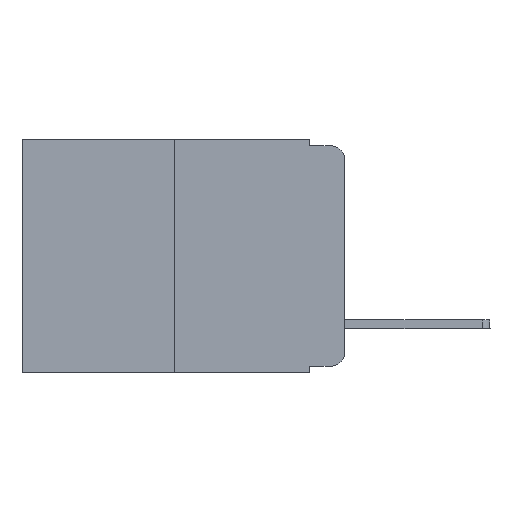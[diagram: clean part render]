
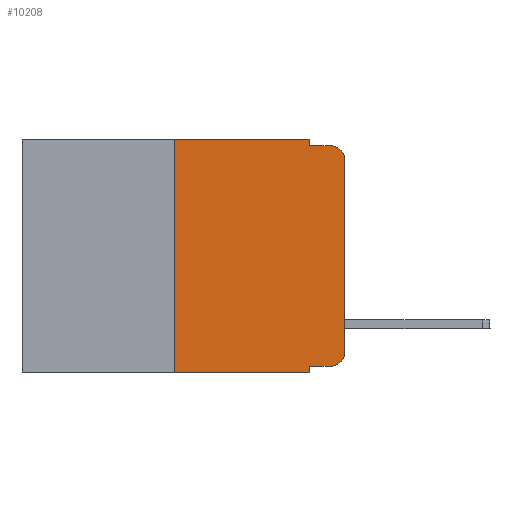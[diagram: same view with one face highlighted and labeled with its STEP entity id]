
A CAD part, left-side view. The second image highlights one B-rep face of the part: STEP entity #10208.
In plain terms, the highlighted planar face has unit normal (-1, 0, 0).
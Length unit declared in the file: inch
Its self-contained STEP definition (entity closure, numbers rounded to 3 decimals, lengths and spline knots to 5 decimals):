
#117 = ORIENTED_EDGE ( 'NONE', *, *, #11305, .F. ) ;
#152 = EDGE_CURVE ( 'NONE', #15001, #13935, #11804, .T. ) ;
#544 = DIRECTION ( 'NONE',  ( 1., 0., 0. ) ) ;
#600 = VECTOR ( 'NONE', #2760, 39.37008 ) ;
#663 = LINE ( 'NONE', #4531, #10908 ) ;
#776 = DIRECTION ( 'NONE',  ( 0., 0., -1. ) ) ;
#1901 = CARTESIAN_POINT ( 'NONE',  ( 0., 0., 0. ) ) ;
#1989 = ORIENTED_EDGE ( 'NONE', *, *, #4190, .F. ) ;
#2088 = VECTOR ( 'NONE', #3190, 39.37008 ) ;
#2105 = CARTESIAN_POINT ( 'NONE',  ( 0., 0.02, -0.333 ) ) ;
#2259 = DIRECTION ( 'NONE',  ( 0., 0., -1. ) ) ;
#2368 = EDGE_CURVE ( 'NONE', #13935, #14282, #10177, .T. ) ;
#2760 = DIRECTION ( 'NONE',  ( 0., -1., 0. ) ) ;
#3080 = DIRECTION ( 'NONE',  ( 0., -1., 0. ) ) ;
#3178 = CARTESIAN_POINT ( 'NONE',  ( 0., 0.051, -0.01 ) ) ;
#3190 = DIRECTION ( 'NONE',  ( 0., 0., 1. ) ) ;
#3295 = AXIS2_PLACEMENT_3D ( 'NONE', #12212, #544, #7604 ) ;
#3315 = DIRECTION ( 'NONE',  ( -1., 0., 0. ) ) ;
#3701 = DIRECTION ( 'NONE',  ( 0., -1., 0. ) ) ;
#3874 = LINE ( 'NONE', #14139, #8647 ) ;
#3954 = CARTESIAN_POINT ( 'NONE',  ( 0., 0.02, -0.313 ) ) ;
#3970 = VERTEX_POINT ( 'NONE', #12723 ) ;
#4188 = CARTESIAN_POINT ( 'NONE',  ( 0., 0., -0.03 ) ) ;
#4190 = EDGE_CURVE ( 'NONE', #8089, #15041, #3874, .T. ) ;
#4531 = CARTESIAN_POINT ( 'NONE',  ( 0., 0.051, -0.333 ) ) ;
#4806 = EDGE_LOOP ( 'NONE', ( #10982, #14694, #13483, #117, #1989, #8035, #8847, #6361, #5822, #6725 ) ) ;
#4891 = CARTESIAN_POINT ( 'NONE',  ( 0., 0.051, -0.333 ) ) ;
#5037 = VERTEX_POINT ( 'NONE', #11154 ) ;
#5162 = CARTESIAN_POINT ( 'NONE',  ( 0., 0., -0.313 ) ) ;
#5822 = ORIENTED_EDGE ( 'NONE', *, *, #9663, .T. ) ;
#6361 = ORIENTED_EDGE ( 'NONE', *, *, #8307, .F. ) ;
#6587 = VERTEX_POINT ( 'NONE', #4891 ) ;
#6725 = ORIENTED_EDGE ( 'NONE', *, *, #10266, .T. ) ;
#7424 = CARTESIAN_POINT ( 'NONE',  ( 0., 0.051, 0. ) ) ;
#7555 = LINE ( 'NONE', #9682, #600 ) ;
#7604 = DIRECTION ( 'NONE',  ( 0., 0., -1. ) ) ;
#7676 = CARTESIAN_POINT ( 'NONE',  ( 0., 0.25, 0. ) ) ;
#7775 = EDGE_CURVE ( 'NONE', #3970, #14282, #10199, .T. ) ;
#7978 = CARTESIAN_POINT ( 'NONE',  ( 0., 0.02, -0.03 ) ) ;
#8035 = ORIENTED_EDGE ( 'NONE', *, *, #8116, .F. ) ;
#8089 = VERTEX_POINT ( 'NONE', #10815 ) ;
#8116 = EDGE_CURVE ( 'NONE', #5037, #8089, #9579, .T. ) ;
#8186 = VECTOR ( 'NONE', #776, 39.37008 ) ;
#8307 = EDGE_CURVE ( 'NONE', #6587, #9195, #10215, .T. ) ;
#8647 = VECTOR ( 'NONE', #3701, 39.37008 ) ;
#8847 = ORIENTED_EDGE ( 'NONE', *, *, #11317, .T. ) ;
#9195 = VERTEX_POINT ( 'NONE', #14285 ) ;
#9216 = AXIS2_PLACEMENT_3D ( 'NONE', #7978, #3315, #9577 ) ;
#9450 = VECTOR ( 'NONE', #3080, 39.37008 ) ;
#9577 = DIRECTION ( 'NONE',  ( 0., 0., -1. ) ) ;
#9579 = LINE ( 'NONE', #7676, #10447 ) ;
#9663 = EDGE_CURVE ( 'NONE', #6587, #13507, #663, .T. ) ;
#9682 = CARTESIAN_POINT ( 'NONE',  ( 0., 0.473, -0.343 ) ) ;
#9775 = DIRECTION ( 'NONE',  ( 0., 0., -1. ) ) ;
#10092 = AXIS2_PLACEMENT_3D ( 'NONE', #3954, #13578, #2259 ) ;
#10177 = CIRCLE ( 'NONE', #9216, 0.02 ) ;
#10199 = LINE ( 'NONE', #3178, #9450 ) ;
#10208 = ADVANCED_FACE ( 'NONE', ( #12166 ), #14593, .F. ) ;
#10215 = LINE ( 'NONE', #13663, #8186 ) ;
#10266 = EDGE_CURVE ( 'NONE', #13507, #15001, #13806, .T. ) ;
#10316 = DIRECTION ( 'NONE',  ( 0., -1., 0. ) ) ;
#10447 = VECTOR ( 'NONE', #13553, 39.37008 ) ;
#10682 = LINE ( 'NONE', #7424, #14307 ) ;
#10756 = CARTESIAN_POINT ( 'NONE',  ( 0., 0.02, -0.01 ) ) ;
#10815 = CARTESIAN_POINT ( 'NONE',  ( 0., 0.25, 0. ) ) ;
#10908 = VECTOR ( 'NONE', #10316, 39.37008 ) ;
#10982 = ORIENTED_EDGE ( 'NONE', *, *, #152, .T. ) ;
#11154 = CARTESIAN_POINT ( 'NONE',  ( 0., 0.25, -0.343 ) ) ;
#11305 = EDGE_CURVE ( 'NONE', #15041, #3970, #10682, .T. ) ;
#11317 = EDGE_CURVE ( 'NONE', #5037, #9195, #7555, .T. ) ;
#11804 = LINE ( 'NONE', #1901, #2088 ) ;
#12166 = FACE_OUTER_BOUND ( 'NONE', #4806, .T. ) ;
#12206 = CARTESIAN_POINT ( 'NONE',  ( 0., 0.051, 0. ) ) ;
#12212 = CARTESIAN_POINT ( 'NONE',  ( 0., 0.473, 0. ) ) ;
#12723 = CARTESIAN_POINT ( 'NONE',  ( 0., 0.051, -0.01 ) ) ;
#13483 = ORIENTED_EDGE ( 'NONE', *, *, #7775, .F. ) ;
#13507 = VERTEX_POINT ( 'NONE', #2105 ) ;
#13553 = DIRECTION ( 'NONE',  ( 0., 0., 1. ) ) ;
#13578 = DIRECTION ( 'NONE',  ( -1., 0., 0. ) ) ;
#13663 = CARTESIAN_POINT ( 'NONE',  ( 0., 0.051, 0. ) ) ;
#13806 = CIRCLE ( 'NONE', #10092, 0.02 ) ;
#13935 = VERTEX_POINT ( 'NONE', #4188 ) ;
#14139 = CARTESIAN_POINT ( 'NONE',  ( 0., 0.473, 0. ) ) ;
#14282 = VERTEX_POINT ( 'NONE', #10756 ) ;
#14285 = CARTESIAN_POINT ( 'NONE',  ( 0., 0.051, -0.343 ) ) ;
#14307 = VECTOR ( 'NONE', #9775, 39.37008 ) ;
#14593 = PLANE ( 'NONE',  #3295 ) ;
#14694 = ORIENTED_EDGE ( 'NONE', *, *, #2368, .T. ) ;
#15001 = VERTEX_POINT ( 'NONE', #5162 ) ;
#15041 = VERTEX_POINT ( 'NONE', #12206 ) ;
